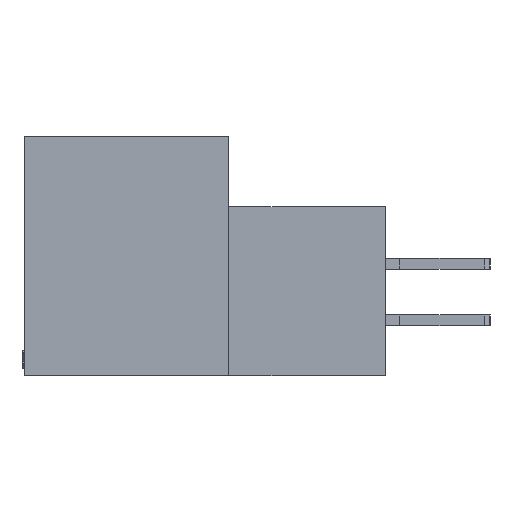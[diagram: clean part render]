
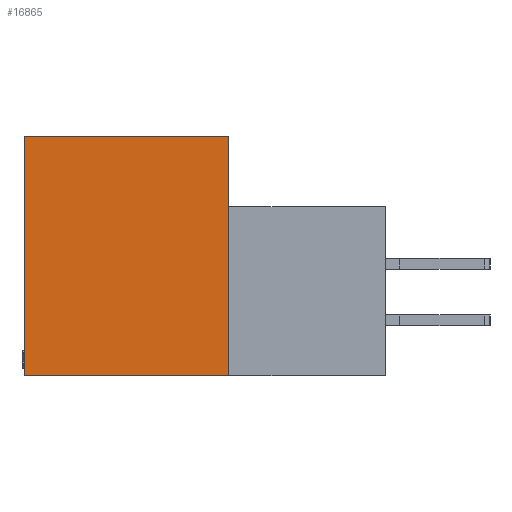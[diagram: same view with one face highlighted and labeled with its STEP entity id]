
A CAD part, left-side view. The second image highlights one B-rep face of the part: STEP entity #16865.
In plain terms, the highlighted planar face has unit normal (-1, 0, 0).
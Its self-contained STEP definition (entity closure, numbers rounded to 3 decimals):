
#1374 = VERTEX_POINT ( 'NONE', #15945 ) ;
#1510 = CARTESIAN_POINT ( 'NONE',  ( 0., 0., 0. ) ) ;
#1843 = FACE_OUTER_BOUND ( 'NONE', #10907, .T. ) ;
#2473 = LINE ( 'NONE', #6196, #22205 ) ;
#3832 = DIRECTION ( 'NONE',  ( 0., 0., -1. ) ) ;
#4438 = DIRECTION ( 'NONE',  ( 0., -1., 0. ) ) ;
#5673 = DIRECTION ( 'NONE',  ( 0., 0., -1. ) ) ;
#6196 = CARTESIAN_POINT ( 'NONE',  ( 0., 0., 0. ) ) ;
#6788 = CARTESIAN_POINT ( 'NONE',  ( 0., 11.506, 0. ) ) ;
#7383 = VECTOR ( 'NONE', #19157, 1000. ) ;
#9008 = VERTEX_POINT ( 'NONE', #21800 ) ;
#10072 = EDGE_CURVE ( 'NONE', #20537, #1374, #19679, .T. ) ;
#10907 = EDGE_LOOP ( 'NONE', ( #14865, #22580, #11124, #21582 ) ) ;
#11124 = ORIENTED_EDGE ( 'NONE', *, *, #22001, .F. ) ;
#12734 = DIRECTION ( 'NONE',  ( 1., 0., 0. ) ) ;
#13303 = VECTOR ( 'NONE', #4438, 1000. ) ;
#14619 = CARTESIAN_POINT ( 'NONE',  ( 0., -8.814, -13.487 ) ) ;
#14673 = EDGE_CURVE ( 'NONE', #1374, #18214, #18035, .T. ) ;
#14865 = ORIENTED_EDGE ( 'NONE', *, *, #10072, .F. ) ;
#15444 = VECTOR ( 'NONE', #28314, 1000. ) ;
#15945 = CARTESIAN_POINT ( 'NONE',  ( 0., 11.506, -13.487 ) ) ;
#16865 = ADVANCED_FACE ( 'NONE', ( #1843 ), #24003, .F. ) ;
#18035 = LINE ( 'NONE', #19259, #7383 ) ;
#18214 = VERTEX_POINT ( 'NONE', #27756 ) ;
#18384 = EDGE_CURVE ( 'NONE', #9008, #20537, #2473, .T. ) ;
#19157 = DIRECTION ( 'NONE',  ( 0., 0., 1. ) ) ;
#19259 = CARTESIAN_POINT ( 'NONE',  ( 0., 11.506, -13.487 ) ) ;
#19679 = LINE ( 'NONE', #14619, #15444 ) ;
#20044 = LINE ( 'NONE', #6788, #13303 ) ;
#20537 = VERTEX_POINT ( 'NONE', #28629 ) ;
#21582 = ORIENTED_EDGE ( 'NONE', *, *, #14673, .F. ) ;
#21800 = CARTESIAN_POINT ( 'NONE',  ( 0., 0., 0. ) ) ;
#22001 = EDGE_CURVE ( 'NONE', #18214, #9008, #20044, .T. ) ;
#22205 = VECTOR ( 'NONE', #3832, 1000. ) ;
#22580 = ORIENTED_EDGE ( 'NONE', *, *, #18384, .F. ) ;
#24003 = PLANE ( 'NONE',  #24813 ) ;
#24813 = AXIS2_PLACEMENT_3D ( 'NONE', #1510, #12734, #5673 ) ;
#27756 = CARTESIAN_POINT ( 'NONE',  ( 0., 11.506, 0. ) ) ;
#28314 = DIRECTION ( 'NONE',  ( 0., 1., 0. ) ) ;
#28629 = CARTESIAN_POINT ( 'NONE',  ( 0., 0., -13.487 ) ) ;
